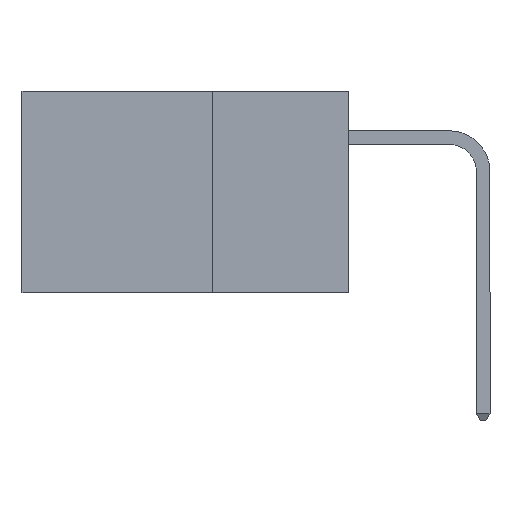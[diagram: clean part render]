
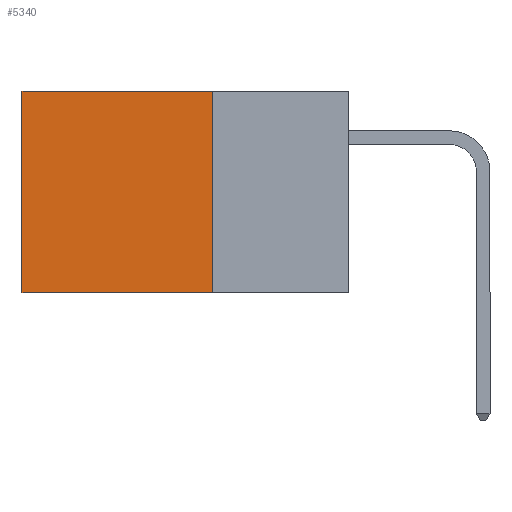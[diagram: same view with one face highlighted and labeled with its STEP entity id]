
A CAD part, left-side view. The second image highlights one B-rep face of the part: STEP entity #5340.
In plain terms, the highlighted planar face has unit normal (-1, 0, 0).
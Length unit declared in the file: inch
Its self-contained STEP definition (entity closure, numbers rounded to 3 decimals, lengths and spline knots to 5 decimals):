
#11 = CARTESIAN_POINT ( 'NONE',  ( 0.2875, 0.25, -0.37 ) ) ;
#711 = CARTESIAN_POINT ( 'NONE',  ( 0.2875, 0.6, 0. ) ) ;
#754 = LINE ( 'NONE', #3425, #7775 ) ;
#836 = LINE ( 'NONE', #2657, #4144 ) ;
#870 = EDGE_CURVE ( 'NONE', #1365, #2422, #6331, .T. ) ;
#1284 = DIRECTION ( 'NONE',  ( 0., 0., -1. ) ) ;
#1365 = VERTEX_POINT ( 'NONE', #11 ) ;
#1405 = EDGE_CURVE ( 'NONE', #7454, #1867, #754, .T. ) ;
#1837 = CARTESIAN_POINT ( 'NONE',  ( 0.2875, 0.25, 0. ) ) ;
#1867 = VERTEX_POINT ( 'NONE', #711 ) ;
#1902 = FACE_OUTER_BOUND ( 'NONE', #4649, .T. ) ;
#2005 = PLANE ( 'NONE',  #3993 ) ;
#2422 = VERTEX_POINT ( 'NONE', #3132 ) ;
#2657 = CARTESIAN_POINT ( 'NONE',  ( 0.2875, 0.6, 0. ) ) ;
#2727 = CARTESIAN_POINT ( 'NONE',  ( 0.2875, 0.25, 0. ) ) ;
#2763 = DIRECTION ( 'NONE',  ( 1., 0., 0. ) ) ;
#2894 = VECTOR ( 'NONE', #1284, 39.37008 ) ;
#3108 = EDGE_CURVE ( 'NONE', #7454, #1365, #6572, .T. ) ;
#3132 = CARTESIAN_POINT ( 'NONE',  ( 0.2875, 0.6, -0.37 ) ) ;
#3425 = CARTESIAN_POINT ( 'NONE',  ( 0.2875, 0.25, 0. ) ) ;
#3537 = DIRECTION ( 'NONE',  ( 0., 1., 0. ) ) ;
#3539 = ORIENTED_EDGE ( 'NONE', *, *, #3108, .F. ) ;
#3554 = CARTESIAN_POINT ( 'NONE',  ( 0.2875, 0.25, 0. ) ) ;
#3680 = CARTESIAN_POINT ( 'NONE',  ( 0.2875, 0.25, -0.37 ) ) ;
#3993 = AXIS2_PLACEMENT_3D ( 'NONE', #2727, #2763, #7315 ) ;
#4144 = VECTOR ( 'NONE', #6000, 39.37008 ) ;
#4649 = EDGE_LOOP ( 'NONE', ( #4660, #7683, #3539, #6127 ) ) ;
#4660 = ORIENTED_EDGE ( 'NONE', *, *, #7496, .T. ) ;
#5340 = ADVANCED_FACE ( 'NONE', ( #1902 ), #2005, .F. ) ;
#6000 = DIRECTION ( 'NONE',  ( 0., 0., -1. ) ) ;
#6127 = ORIENTED_EDGE ( 'NONE', *, *, #1405, .T. ) ;
#6211 = DIRECTION ( 'NONE',  ( 0., 1., 0. ) ) ;
#6331 = LINE ( 'NONE', #3680, #8335 ) ;
#6572 = LINE ( 'NONE', #3554, #2894 ) ;
#7315 = DIRECTION ( 'NONE',  ( 0., 0., -1. ) ) ;
#7454 = VERTEX_POINT ( 'NONE', #1837 ) ;
#7496 = EDGE_CURVE ( 'NONE', #1867, #2422, #836, .T. ) ;
#7683 = ORIENTED_EDGE ( 'NONE', *, *, #870, .F. ) ;
#7775 = VECTOR ( 'NONE', #6211, 39.37008 ) ;
#8335 = VECTOR ( 'NONE', #3537, 39.37008 ) ;
